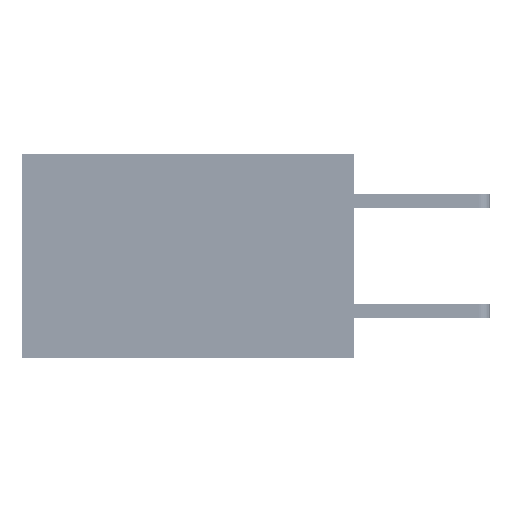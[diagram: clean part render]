
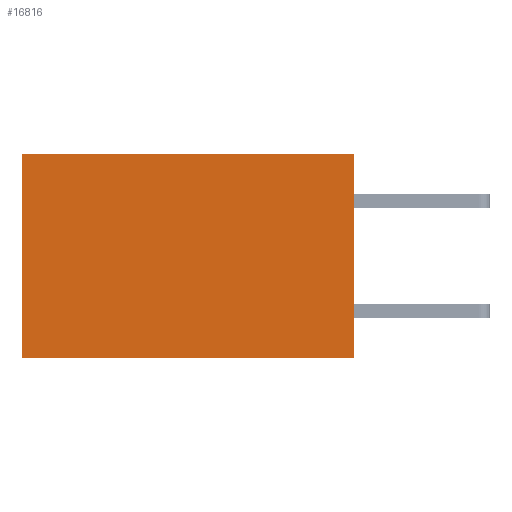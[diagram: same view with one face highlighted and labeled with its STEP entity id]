
A CAD part, left-side view. The second image highlights one B-rep face of the part: STEP entity #16816.
In plain terms, the highlighted planar face has unit normal (-1, 0, 0).
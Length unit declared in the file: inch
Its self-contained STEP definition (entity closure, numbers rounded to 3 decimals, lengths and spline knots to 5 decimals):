
#1245 = ORIENTED_EDGE ( 'NONE', *, *, #24592, .T. ) ;
#1875 = CARTESIAN_POINT ( 'NONE',  ( 0.2875, 0., -0.37 ) ) ;
#4346 = EDGE_CURVE ( 'NONE', #10658, #49570, #42053, .T. ) ;
#8757 = ORIENTED_EDGE ( 'NONE', *, *, #12480, .F. ) ;
#9820 = VECTOR ( 'NONE', #50998, 39.37008 ) ;
#10658 = VERTEX_POINT ( 'NONE', #14400 ) ;
#12480 = EDGE_CURVE ( 'NONE', #49027, #49570, #25383, .T. ) ;
#13618 = VECTOR ( 'NONE', #38834, 39.37008 ) ;
#14400 = CARTESIAN_POINT ( 'NONE',  ( 0.2875, 0.6, 0. ) ) ;
#16816 = ADVANCED_FACE ( 'NONE', ( #17633 ), #48923, .F. ) ;
#17042 = LINE ( 'NONE', #36586, #19104 ) ;
#17633 = FACE_OUTER_BOUND ( 'NONE', #33556, .T. ) ;
#18336 = DIRECTION ( 'NONE',  ( 0., 0., -1. ) ) ;
#18585 = CARTESIAN_POINT ( 'NONE',  ( 0.2875, 0.6, 0. ) ) ;
#19104 = VECTOR ( 'NONE', #32937, 39.37008 ) ;
#22688 = EDGE_CURVE ( 'NONE', #39036, #49027, #36126, .T. ) ;
#24592 = EDGE_CURVE ( 'NONE', #39036, #10658, #17042, .T. ) ;
#25383 = LINE ( 'NONE', #49115, #13618 ) ;
#27274 = ORIENTED_EDGE ( 'NONE', *, *, #4346, .T. ) ;
#32760 = DIRECTION ( 'NONE',  ( 0., 0., -1. ) ) ;
#32937 = DIRECTION ( 'NONE',  ( 0., 1., 0. ) ) ;
#33556 = EDGE_LOOP ( 'NONE', ( #27274, #8757, #49133, #1245 ) ) ;
#36126 = LINE ( 'NONE', #47333, #9820 ) ;
#36586 = CARTESIAN_POINT ( 'NONE',  ( 0.2875, 0., 0. ) ) ;
#36670 = CARTESIAN_POINT ( 'NONE',  ( 0.2875, 0., 0. ) ) ;
#37042 = CARTESIAN_POINT ( 'NONE',  ( 0.2875, 0., 0. ) ) ;
#38834 = DIRECTION ( 'NONE',  ( 0., 1., 0. ) ) ;
#39036 = VERTEX_POINT ( 'NONE', #37042 ) ;
#42053 = LINE ( 'NONE', #18585, #50408 ) ;
#43670 = AXIS2_PLACEMENT_3D ( 'NONE', #36670, #49442, #32760 ) ;
#47333 = CARTESIAN_POINT ( 'NONE',  ( 0.2875, 0., 0. ) ) ;
#48923 = PLANE ( 'NONE',  #43670 ) ;
#49027 = VERTEX_POINT ( 'NONE', #1875 ) ;
#49115 = CARTESIAN_POINT ( 'NONE',  ( 0.2875, 0., -0.37 ) ) ;
#49133 = ORIENTED_EDGE ( 'NONE', *, *, #22688, .F. ) ;
#49442 = DIRECTION ( 'NONE',  ( 1., 0., 0. ) ) ;
#49570 = VERTEX_POINT ( 'NONE', #50019 ) ;
#50019 = CARTESIAN_POINT ( 'NONE',  ( 0.2875, 0.6, -0.37 ) ) ;
#50408 = VECTOR ( 'NONE', #18336, 39.37008 ) ;
#50998 = DIRECTION ( 'NONE',  ( 0., 0., -1. ) ) ;
